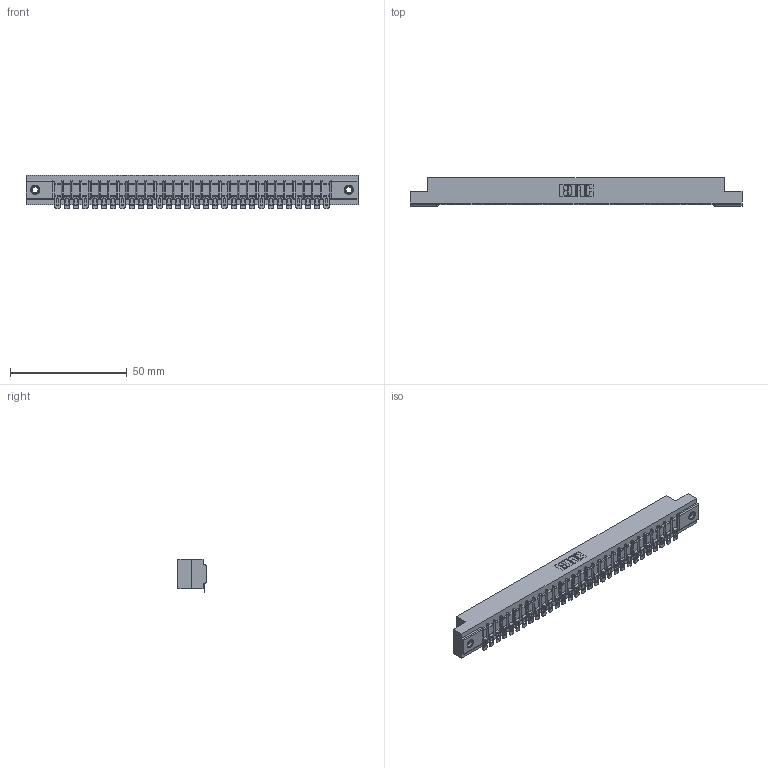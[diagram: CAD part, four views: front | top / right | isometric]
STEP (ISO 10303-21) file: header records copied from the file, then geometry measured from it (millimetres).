
FILE_DESCRIPTION (( 'STEP AP203' ), '1' );
FILE_NAME ('307-030-454-107.STEP', '2020-09-28T12:13:16', ( '' ), ( '' ), 'SwSTEP 2.0', 'SolidWorks 2020', '' );
FILE_SCHEMA (( 'CONFIG_CONTROL_DESIGN' ));
Length unit declared in the file: inch
Products named in the file (4): 345-250-001_345-250-005-103; 307 Part_.156 Dia Mounting Holes; 307-290-002_554; 307-030-454-107
Assembly tree (33 placements, depth 2):
  307-030-454-107
    307 Part_.156 Dia Mounting Holes
    307-290-002_554  x30
    345-250-001_345-250-005-103  x2
Bounding box: 141.88 x 12.01 x 14.52 mm (x, y, z)
Volume: 15091.2 mm3; surface area: 18860.5 mm2
Topology: 33 solids, 33 shells, 2639 faces, 8049 edges, 5274 vertices
Faces by surface type: plane 1482, cylinder 1079, sphere 62, cone 12, torus 4
Entity records: 29348 total; most frequent: CARTESIAN_POINT 4929, ORIENTED_EDGE 4912, DIRECTION 4810, EDGE_CURVE 2456, LINE 1868, VECTOR 1868, VERTEX_POINT 1590, AXIS2_PLACEMENT_3D 1471
